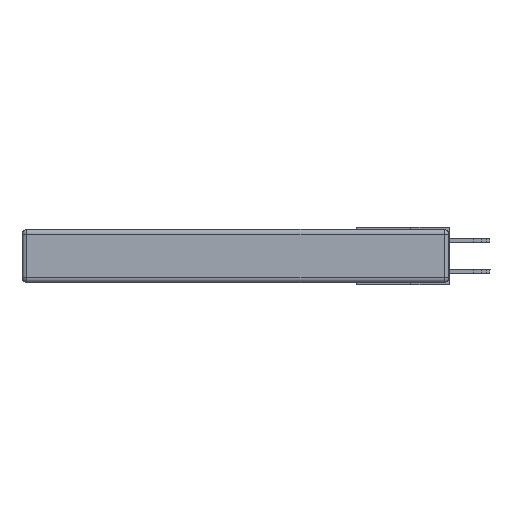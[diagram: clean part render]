
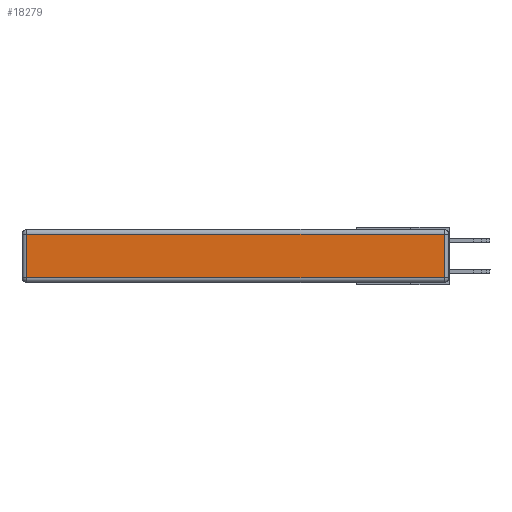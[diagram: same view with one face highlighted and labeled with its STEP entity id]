
A CAD part, left-side view. The second image highlights one B-rep face of the part: STEP entity #18279.
In plain terms, the highlighted planar face has unit normal (-1, 0, 0).
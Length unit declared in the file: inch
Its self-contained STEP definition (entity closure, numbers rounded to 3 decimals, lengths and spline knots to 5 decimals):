
#238 = EDGE_CURVE ( 'NONE', #7189, #16480, #6401, .T. ) ;
#935 = DIRECTION ( 'NONE',  ( 0., -1., 0. ) ) ;
#3593 = CARTESIAN_POINT ( 'NONE',  ( 0., 0., -0.343 ) ) ;
#4196 = VERTEX_POINT ( 'NONE', #17688 ) ;
#4788 = EDGE_CURVE ( 'NONE', #16480, #4196, #5264, .T. ) ;
#4916 = FACE_OUTER_BOUND ( 'NONE', #15993, .T. ) ;
#5123 = DIRECTION ( 'NONE',  ( 0., 0., 1. ) ) ;
#5264 = LINE ( 'NONE', #17461, #7643 ) ;
#5419 = DIRECTION ( 'NONE',  ( 0., 1., 0. ) ) ;
#6204 = VECTOR ( 'NONE', #7486, 39.37008 ) ;
#6401 = LINE ( 'NONE', #16140, #10916 ) ;
#6415 = EDGE_CURVE ( 'NONE', #4196, #14548, #8301, .T. ) ;
#6456 = ORIENTED_EDGE ( 'NONE', *, *, #16709, .T. ) ;
#7189 = VERTEX_POINT ( 'NONE', #13280 ) ;
#7486 = DIRECTION ( 'NONE',  ( 0., 0., -1. ) ) ;
#7643 = VECTOR ( 'NONE', #5123, 39.37008 ) ;
#8301 = LINE ( 'NONE', #12440, #14220 ) ;
#9067 = LINE ( 'NONE', #13597, #6204 ) ;
#9098 = ORIENTED_EDGE ( 'NONE', *, *, #6415, .T. ) ;
#10727 = CARTESIAN_POINT ( 'NONE',  ( 0., 2.72, -0.03 ) ) ;
#10916 = VECTOR ( 'NONE', #935, 39.37008 ) ;
#11633 = DIRECTION ( 'NONE',  ( 0., 0., 1. ) ) ;
#12329 = ORIENTED_EDGE ( 'NONE', *, *, #4788, .T. ) ;
#12440 = CARTESIAN_POINT ( 'NONE',  ( 0., 2.75, -0.03 ) ) ;
#13280 = CARTESIAN_POINT ( 'NONE',  ( 0., 2.72, -0.313 ) ) ;
#13597 = CARTESIAN_POINT ( 'NONE',  ( 0., 2.72, -0.343 ) ) ;
#14220 = VECTOR ( 'NONE', #5419, 39.37008 ) ;
#14242 = DIRECTION ( 'NONE',  ( -1., 0., 0. ) ) ;
#14548 = VERTEX_POINT ( 'NONE', #10727 ) ;
#14628 = CARTESIAN_POINT ( 'NONE',  ( 0., 0.03, -0.313 ) ) ;
#15898 = ORIENTED_EDGE ( 'NONE', *, *, #238, .T. ) ;
#15993 = EDGE_LOOP ( 'NONE', ( #15898, #12329, #9098, #6456 ) ) ;
#16140 = CARTESIAN_POINT ( 'NONE',  ( 0., 0., -0.313 ) ) ;
#16480 = VERTEX_POINT ( 'NONE', #14628 ) ;
#16709 = EDGE_CURVE ( 'NONE', #14548, #7189, #9067, .T. ) ;
#16816 = AXIS2_PLACEMENT_3D ( 'NONE', #3593, #14242, #11633 ) ;
#17461 = CARTESIAN_POINT ( 'NONE',  ( 0., 0.03, -0.343 ) ) ;
#17688 = CARTESIAN_POINT ( 'NONE',  ( 0., 0.03, -0.03 ) ) ;
#18279 = ADVANCED_FACE ( 'NONE', ( #4916 ), #18891, .T. ) ;
#18891 = PLANE ( 'NONE',  #16816 ) ;
